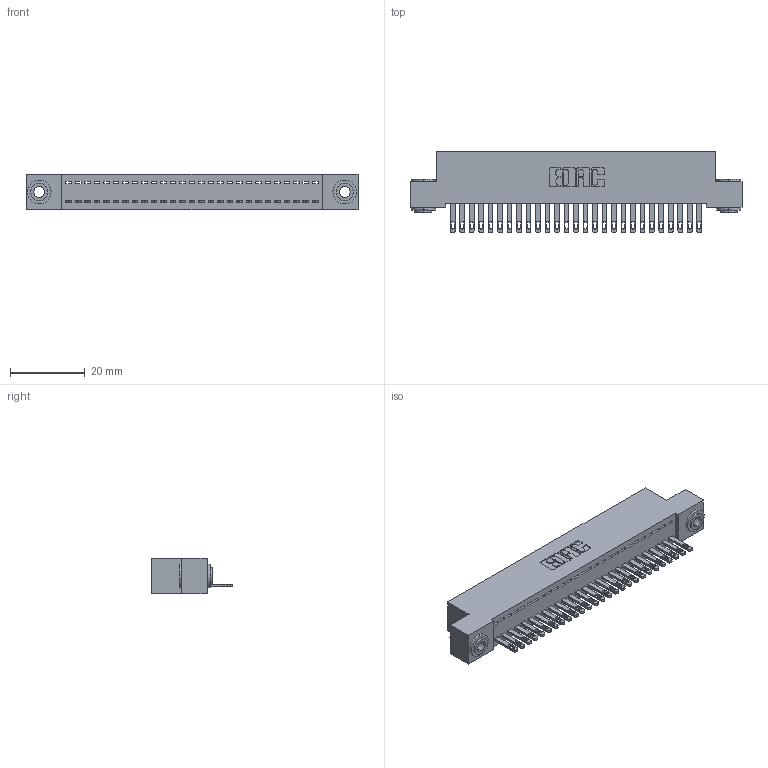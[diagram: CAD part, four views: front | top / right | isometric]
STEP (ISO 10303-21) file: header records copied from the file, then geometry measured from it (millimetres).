
FILE_DESCRIPTION (( 'STEP AP203' ), '1' );
FILE_NAME ('892-027-500-103.STEP', '2020-09-21T14:45:22', ( '' ), ( '' ), 'SwSTEP 2.0', 'SolidWorks 2020', '' );
FILE_SCHEMA (( 'CONFIG_CONTROL_DESIGN' ));
Length unit declared in the file: inch
Products named in the file (4): 842 Part_.156 TH; 345-292-001_345-293-100; 892-027-500-103; 342-250-002_345-250-002-102
Assembly tree (30 placements, depth 2):
  892-027-500-103
    842 Part_.156 TH
    345-292-001_345-293-100  x27
    342-250-002_345-250-002-102  x2
Bounding box: 88.9 x 21.85 x 9.4 mm (x, y, z)
Volume: 7779 mm3; surface area: 11422.4 mm2
Topology: 30 solids, 30 shells, 1606 faces, 4911 edges, 3270 vertices
Faces by surface type: plane 1048, cylinder 550, cone 8
Entity records: 18894 total; most frequent: CARTESIAN_POINT 3238, ORIENTED_EDGE 3194, DIRECTION 2797, EDGE_CURVE 1597, VECTOR 1441, LINE 1441, VERTEX_POINT 1062, AXIS2_PLACEMENT_3D 678
